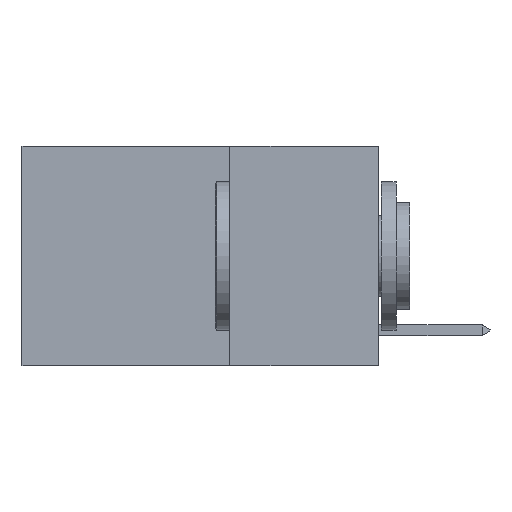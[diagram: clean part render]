
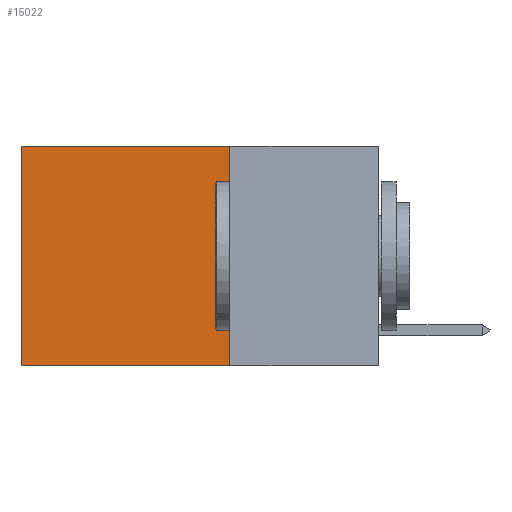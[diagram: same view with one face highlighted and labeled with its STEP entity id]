
A CAD part, left-side view. The second image highlights one B-rep face of the part: STEP entity #15022.
In plain terms, the highlighted planar face has unit normal (-1, 0, 0).
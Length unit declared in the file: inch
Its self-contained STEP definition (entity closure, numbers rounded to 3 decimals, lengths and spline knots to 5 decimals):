
#211 = CARTESIAN_POINT ( 'NONE',  ( 0.2625, 0.25, 0. ) ) ;
#240 = ORIENTED_EDGE ( 'NONE', *, *, #12558, .T. ) ;
#1847 = CARTESIAN_POINT ( 'NONE',  ( 0.2625, 0.25, 0. ) ) ;
#2681 = EDGE_CURVE ( 'NONE', #3202, #10424, #2709, .T. ) ;
#2709 = LINE ( 'NONE', #11906, #7696 ) ;
#3035 = CARTESIAN_POINT ( 'NONE',  ( 0.2625, 0.25, -0.37 ) ) ;
#3167 = VERTEX_POINT ( 'NONE', #19556 ) ;
#3202 = VERTEX_POINT ( 'NONE', #6334 ) ;
#3273 = EDGE_CURVE ( 'NONE', #10424, #7886, #6429, .T. ) ;
#3529 = DIRECTION ( 'NONE',  ( 0., 0., -1. ) ) ;
#3728 = VECTOR ( 'NONE', #6595, 39.37008 ) ;
#3900 = VECTOR ( 'NONE', #8055, 39.37008 ) ;
#4987 = PLANE ( 'NONE',  #10494 ) ;
#5713 = EDGE_LOOP ( 'NONE', ( #240, #7527, #13164, #9504 ) ) ;
#5753 = DIRECTION ( 'NONE',  ( 0., 0., -1. ) ) ;
#6311 = DIRECTION ( 'NONE',  ( 1., 0., 0. ) ) ;
#6334 = CARTESIAN_POINT ( 'NONE',  ( 0.2625, 0.25, 0. ) ) ;
#6429 = LINE ( 'NONE', #6534, #3900 ) ;
#6534 = CARTESIAN_POINT ( 'NONE',  ( 0.2625, 0.25, -0.37 ) ) ;
#6595 = DIRECTION ( 'NONE',  ( 0., 1., 0. ) ) ;
#7527 = ORIENTED_EDGE ( 'NONE', *, *, #3273, .F. ) ;
#7696 = VECTOR ( 'NONE', #5753, 39.37008 ) ;
#7886 = VERTEX_POINT ( 'NONE', #17739 ) ;
#8055 = DIRECTION ( 'NONE',  ( 0., 1., 0. ) ) ;
#9504 = ORIENTED_EDGE ( 'NONE', *, *, #18125, .T. ) ;
#9523 = LINE ( 'NONE', #211, #3728 ) ;
#9618 = CARTESIAN_POINT ( 'NONE',  ( 0.2625, 0.6, 0. ) ) ;
#10424 = VERTEX_POINT ( 'NONE', #3035 ) ;
#10494 = AXIS2_PLACEMENT_3D ( 'NONE', #1847, #6311, #17016 ) ;
#11241 = LINE ( 'NONE', #9618, #18150 ) ;
#11906 = CARTESIAN_POINT ( 'NONE',  ( 0.2625, 0.25, 0. ) ) ;
#12558 = EDGE_CURVE ( 'NONE', #3167, #7886, #11241, .T. ) ;
#13164 = ORIENTED_EDGE ( 'NONE', *, *, #2681, .F. ) ;
#15022 = ADVANCED_FACE ( 'NONE', ( #18727 ), #4987, .F. ) ;
#17016 = DIRECTION ( 'NONE',  ( 0., 0., -1. ) ) ;
#17739 = CARTESIAN_POINT ( 'NONE',  ( 0.2625, 0.6, -0.37 ) ) ;
#18125 = EDGE_CURVE ( 'NONE', #3202, #3167, #9523, .T. ) ;
#18150 = VECTOR ( 'NONE', #3529, 39.37008 ) ;
#18727 = FACE_OUTER_BOUND ( 'NONE', #5713, .T. ) ;
#19556 = CARTESIAN_POINT ( 'NONE',  ( 0.2625, 0.6, 0. ) ) ;
